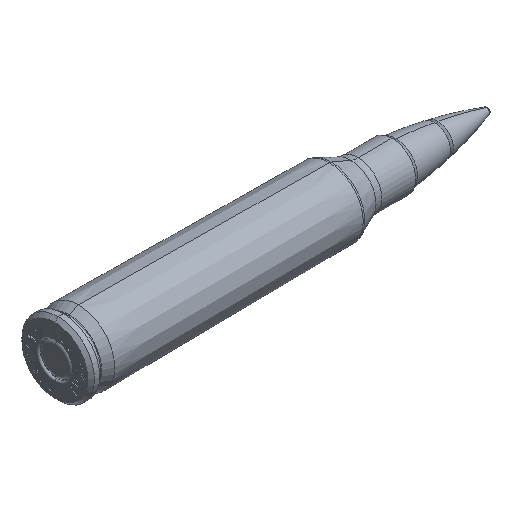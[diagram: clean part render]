
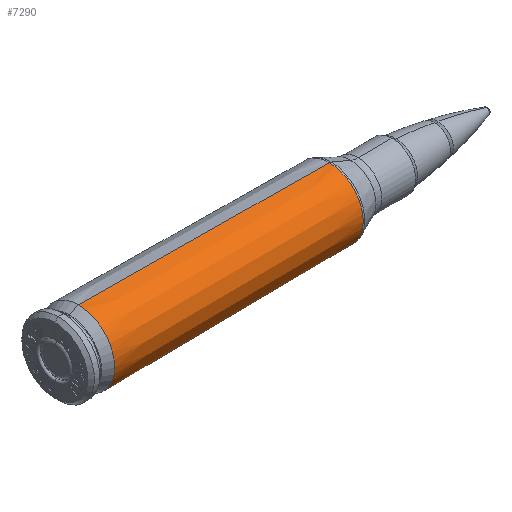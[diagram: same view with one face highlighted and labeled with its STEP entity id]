
A CAD part, isometric view. The second image highlights one B-rep face of the part: STEP entity #7290.
In plain terms, the highlighted conical face has half-angle 0.5 degrees and reference radius 4.801 mm.
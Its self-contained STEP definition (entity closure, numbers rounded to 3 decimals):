
#1083 = CARTESIAN_POINT ( 'NONE',  ( -9.959, 25.85, 31.776 ) ) ;
#3200 = EDGE_LOOP ( 'NONE', ( #24152, #20977, #29328, #26476 ) ) ;
#3439 = DIRECTION ( 'NONE',  ( -1., 0., -0.009 ) ) ;
#4232 = VECTOR ( 'NONE', #3439, 1000. ) ;
#4314 = VERTEX_POINT ( 'NONE', #34952 ) ;
#4473 = FACE_OUTER_BOUND ( 'NONE', #3200, .T. ) ;
#4549 = CIRCLE ( 'NONE', #24815, 4.801 ) ;
#6172 = LINE ( 'NONE', #1083, #4232 ) ;
#7011 = DIRECTION ( 'NONE',  ( 0., 0., 1. ) ) ;
#7290 = ADVANCED_FACE ( 'NONE', ( #4473 ), #31952, .T. ) ;
#8655 = VECTOR ( 'NONE', #15439, 1000. ) ;
#9719 = CARTESIAN_POINT ( 'NONE',  ( -9.959, 25.85, 36.577 ) ) ;
#12002 = VERTEX_POINT ( 'NONE', #13736 ) ;
#13736 = CARTESIAN_POINT ( 'NONE',  ( 23.274, 25.85, 32.066 ) ) ;
#15439 = DIRECTION ( 'NONE',  ( -1., 0., 0.009 ) ) ;
#15801 = LINE ( 'NONE', #24322, #8655 ) ;
#16804 = EDGE_CURVE ( 'NONE', #30004, #33379, #4549, .T. ) ;
#16996 = CIRCLE ( 'NONE', #22186, 4.511 ) ;
#19019 = CARTESIAN_POINT ( 'NONE',  ( -9.959, 25.85, 31.776 ) ) ;
#20977 = ORIENTED_EDGE ( 'NONE', *, *, #23645, .T. ) ;
#22186 = AXIS2_PLACEMENT_3D ( 'NONE', #28045, #28219, #25145 ) ;
#23015 = CARTESIAN_POINT ( 'NONE',  ( -9.959, 25.85, 41.377 ) ) ;
#23645 = EDGE_CURVE ( 'NONE', #12002, #4314, #16996, .T. ) ;
#24152 = ORIENTED_EDGE ( 'NONE', *, *, #27652, .F. ) ;
#24322 = CARTESIAN_POINT ( 'NONE',  ( -9.959, 25.85, 41.377 ) ) ;
#24815 = AXIS2_PLACEMENT_3D ( 'NONE', #31610, #28894, #26179 ) ;
#25145 = DIRECTION ( 'NONE',  ( 0., 0., 1. ) ) ;
#26179 = DIRECTION ( 'NONE',  ( 0., 0., 1. ) ) ;
#26476 = ORIENTED_EDGE ( 'NONE', *, *, #16804, .F. ) ;
#27652 = EDGE_CURVE ( 'NONE', #12002, #30004, #6172, .T. ) ;
#28045 = CARTESIAN_POINT ( 'NONE',  ( 23.274, 25.85, 36.577 ) ) ;
#28219 = DIRECTION ( 'NONE',  ( -1., 0., 0. ) ) ;
#28894 = DIRECTION ( 'NONE',  ( -1., 0., 0. ) ) ;
#29050 = AXIS2_PLACEMENT_3D ( 'NONE', #9719, #31847, #7011 ) ;
#29328 = ORIENTED_EDGE ( 'NONE', *, *, #34029, .T. ) ;
#30004 = VERTEX_POINT ( 'NONE', #19019 ) ;
#31610 = CARTESIAN_POINT ( 'NONE',  ( -9.959, 25.85, 36.577 ) ) ;
#31847 = DIRECTION ( 'NONE',  ( -1., 0., 0. ) ) ;
#31952 = CONICAL_SURFACE ( 'NONE', #29050, 4.801, 0.009 ) ;
#33379 = VERTEX_POINT ( 'NONE', #23015 ) ;
#34029 = EDGE_CURVE ( 'NONE', #4314, #33379, #15801, .T. ) ;
#34952 = CARTESIAN_POINT ( 'NONE',  ( 23.274, 25.85, 41.087 ) ) ;
